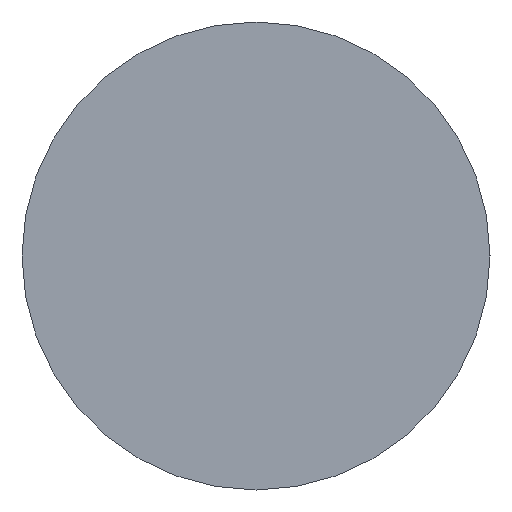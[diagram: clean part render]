
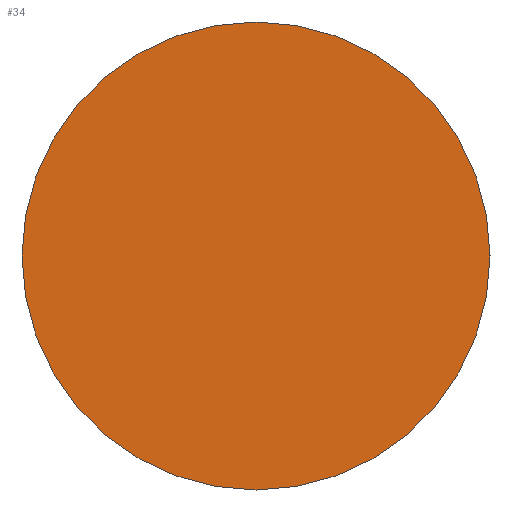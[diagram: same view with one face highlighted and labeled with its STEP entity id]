
A CAD part, left-side view. The second image highlights one B-rep face of the part: STEP entity #34.
In plain terms, the highlighted planar face has unit normal (-1, 0, 0).
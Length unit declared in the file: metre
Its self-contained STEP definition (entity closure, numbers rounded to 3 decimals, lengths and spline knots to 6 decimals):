
#34 = ADVANCED_FACE( '', ( #66 ), #67, .T. );
#66 = FACE_OUTER_BOUND( '', #95, .T. );
#67 = PLANE( '', #96 );
#95 = EDGE_LOOP( '', ( #122 ) );
#96 = AXIS2_PLACEMENT_3D( '', #123, #124, #125 );
#122 = ORIENTED_EDGE( '', *, *, #145, .F. );
#123 = CARTESIAN_POINT( '', ( 0., 0., 0. ) );
#124 = DIRECTION( '', ( -1., 0., 0. ) );
#125 = DIRECTION( '', ( 0., -1., 0. ) );
#145 = EDGE_CURVE( '', #156, #156, #157, .T. );
#156 = VERTEX_POINT( '', #172 );
#157 = CIRCLE( '', #173, 0.00635 );
#172 = CARTESIAN_POINT( '', ( 0., 0.00635, 0. ) );
#173 = AXIS2_PLACEMENT_3D( '', #187, #188, #189 );
#187 = CARTESIAN_POINT( '', ( 0., 0., 0. ) );
#188 = DIRECTION( '', ( 1., 0., 0. ) );
#189 = DIRECTION( '', ( 0., 1., 0. ) );
